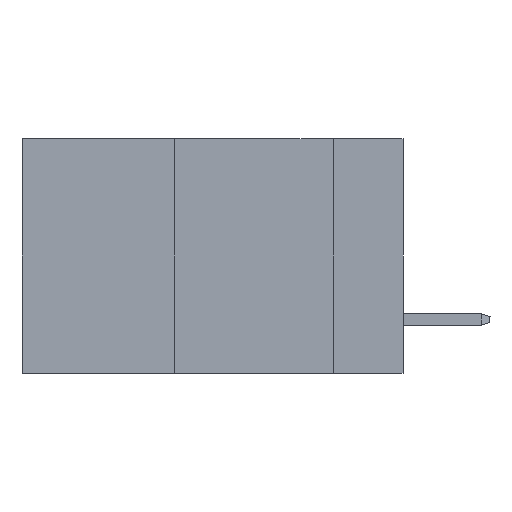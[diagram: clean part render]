
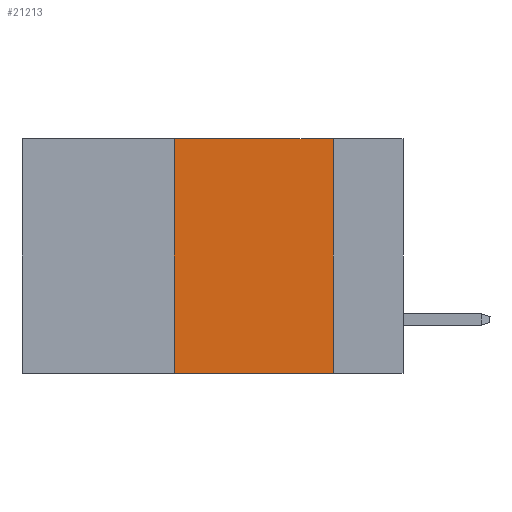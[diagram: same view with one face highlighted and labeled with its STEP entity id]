
A CAD part, left-side view. The second image highlights one B-rep face of the part: STEP entity #21213.
In plain terms, the highlighted planar face has unit normal (-1, 0, 0).
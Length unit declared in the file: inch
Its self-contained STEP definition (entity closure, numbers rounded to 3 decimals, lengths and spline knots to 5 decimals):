
#1133 = CARTESIAN_POINT ( 'NONE',  ( 0., 0.11, 0. ) ) ;
#1174 = VERTEX_POINT ( 'NONE', #9624 ) ;
#2386 = DIRECTION ( 'NONE',  ( 0., 0., -1. ) ) ;
#5656 = LINE ( 'NONE', #10339, #27134 ) ;
#6289 = EDGE_CURVE ( 'NONE', #11063, #11659, #5656, .T. ) ;
#6943 = CARTESIAN_POINT ( 'NONE',  ( 0., 0.36, 0. ) ) ;
#7719 = LINE ( 'NONE', #10224, #25478 ) ;
#9565 = ORIENTED_EDGE ( 'NONE', *, *, #12404, .T. ) ;
#9624 = CARTESIAN_POINT ( 'NONE',  ( 0., 0.11, 0. ) ) ;
#10006 = CARTESIAN_POINT ( 'NONE',  ( 0., 0.36, -0.37 ) ) ;
#10224 = CARTESIAN_POINT ( 'NONE',  ( 0., 0.6, -0.37 ) ) ;
#10339 = CARTESIAN_POINT ( 'NONE',  ( 0., 0.36, 0. ) ) ;
#11063 = VERTEX_POINT ( 'NONE', #10006 ) ;
#11232 = CARTESIAN_POINT ( 'NONE',  ( 0., 0.11, -0.37 ) ) ;
#11659 = VERTEX_POINT ( 'NONE', #6943 ) ;
#11887 = VECTOR ( 'NONE', #25315, 39.37008 ) ;
#12404 = EDGE_CURVE ( 'NONE', #11063, #14535, #7719, .T. ) ;
#13062 = CARTESIAN_POINT ( 'NONE',  ( 0., 0.6, 0. ) ) ;
#13799 = AXIS2_PLACEMENT_3D ( 'NONE', #27802, #29673, #2386 ) ;
#14535 = VERTEX_POINT ( 'NONE', #11232 ) ;
#14952 = LINE ( 'NONE', #13062, #11887 ) ;
#15499 = DIRECTION ( 'NONE',  ( 0., 0., 1. ) ) ;
#17362 = EDGE_CURVE ( 'NONE', #1174, #14535, #21525, .T. ) ;
#19759 = FACE_OUTER_BOUND ( 'NONE', #30028, .T. ) ;
#20600 = ORIENTED_EDGE ( 'NONE', *, *, #17362, .F. ) ;
#21213 = ADVANCED_FACE ( 'NONE', ( #19759 ), #24607, .F. ) ;
#21359 = VECTOR ( 'NONE', #29075, 39.37008 ) ;
#21525 = LINE ( 'NONE', #1133, #21359 ) ;
#24607 = PLANE ( 'NONE',  #13799 ) ;
#25315 = DIRECTION ( 'NONE',  ( 0., -1., 0. ) ) ;
#25478 = VECTOR ( 'NONE', #32653, 39.37008 ) ;
#25606 = ORIENTED_EDGE ( 'NONE', *, *, #6289, .F. ) ;
#27134 = VECTOR ( 'NONE', #15499, 39.37008 ) ;
#27533 = EDGE_CURVE ( 'NONE', #11659, #1174, #14952, .T. ) ;
#27802 = CARTESIAN_POINT ( 'NONE',  ( 0., 0.6, 0. ) ) ;
#29075 = DIRECTION ( 'NONE',  ( 0., 0., -1. ) ) ;
#29673 = DIRECTION ( 'NONE',  ( 1., 0., 0. ) ) ;
#30028 = EDGE_LOOP ( 'NONE', ( #20600, #31799, #25606, #9565 ) ) ;
#31799 = ORIENTED_EDGE ( 'NONE', *, *, #27533, .F. ) ;
#32653 = DIRECTION ( 'NONE',  ( 0., -1., 0. ) ) ;
